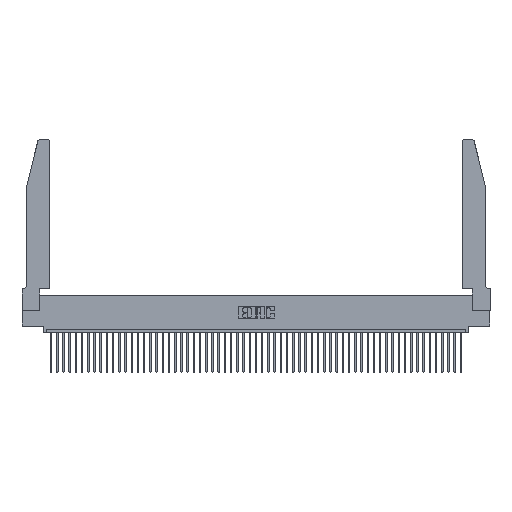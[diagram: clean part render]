
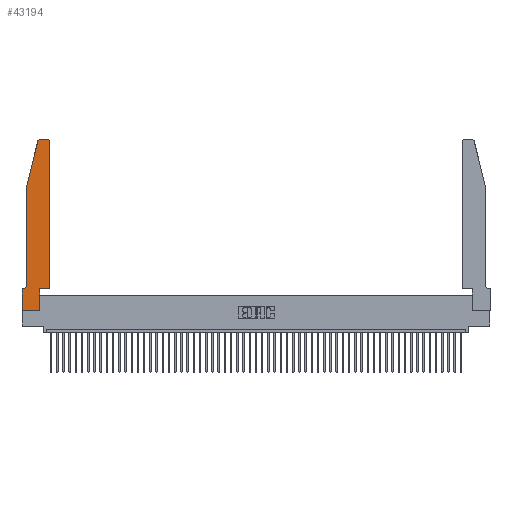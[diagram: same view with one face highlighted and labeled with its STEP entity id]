
A CAD part, top view. The second image highlights one B-rep face of the part: STEP entity #43194.
In plain terms, the highlighted planar face has unit normal (0, 0, 1).
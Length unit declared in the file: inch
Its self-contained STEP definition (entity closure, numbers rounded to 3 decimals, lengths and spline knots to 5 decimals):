
#188 = EDGE_LOOP ( 'NONE', ( #15539, #263, #4675, #17371, #25814, #16195, #5361, #44712, #41587, #32840, #48203, #21301 ) ) ;
#263 = ORIENTED_EDGE ( 'NONE', *, *, #28175, .T. ) ;
#366 = VERTEX_POINT ( 'NONE', #3941 ) ;
#711 = DIRECTION ( 'NONE',  ( 1., 0., 0. ) ) ;
#1036 = CARTESIAN_POINT ( 'NONE',  ( 0.4505, 0.35, 0.37 ) ) ;
#1436 = AXIS2_PLACEMENT_3D ( 'NONE', #32717, #16441, #5233 ) ;
#1506 = VERTEX_POINT ( 'NONE', #40229 ) ;
#2761 = CARTESIAN_POINT ( 'NONE',  ( 0.2865, 0.35, 0.37 ) ) ;
#3041 = VECTOR ( 'NONE', #23626, 39.37008 ) ;
#3048 = CARTESIAN_POINT ( 'NONE',  ( 0., 0.35, 0.37 ) ) ;
#3309 = VERTEX_POINT ( 'NONE', #19532 ) ;
#3941 = CARTESIAN_POINT ( 'NONE',  ( 0.2865, 0., 0.37 ) ) ;
#4309 = LINE ( 'NONE', #30593, #48179 ) ;
#4675 = ORIENTED_EDGE ( 'NONE', *, *, #12563, .T. ) ;
#5233 = DIRECTION ( 'NONE',  ( 1., 0., 0. ) ) ;
#5361 = ORIENTED_EDGE ( 'NONE', *, *, #14542, .T. ) ;
#6517 = LINE ( 'NONE', #10998, #42180 ) ;
#7146 = AXIS2_PLACEMENT_3D ( 'NONE', #3048, #35055, #39595 ) ;
#7967 = CARTESIAN_POINT ( 'NONE',  ( 0.2605, 2.75, 0.37 ) ) ;
#8789 = DIRECTION ( 'NONE',  ( 0., 1., 0. ) ) ;
#10096 = LINE ( 'NONE', #45011, #44548 ) ;
#10459 = DIRECTION ( 'NONE',  ( 0., 1., 0. ) ) ;
#10569 = AXIS2_PLACEMENT_3D ( 'NONE', #41142, #24911, #16986 ) ;
#10998 = CARTESIAN_POINT ( 'NONE',  ( 0.0755, 0.35, 0.37 ) ) ;
#11229 = CARTESIAN_POINT ( 'NONE',  ( 0.25487, 2.72718, 0.37 ) ) ;
#12563 = EDGE_CURVE ( 'NONE', #13031, #3309, #36550, .T. ) ;
#13031 = VERTEX_POINT ( 'NONE', #11229 ) ;
#13241 = EDGE_CURVE ( 'NONE', #15223, #44950, #6517, .T. ) ;
#13855 = LINE ( 'NONE', #7967, #19550 ) ;
#14542 = EDGE_CURVE ( 'NONE', #44950, #41553, #10096, .T. ) ;
#14568 = PLANE ( 'NONE',  #7146 ) ;
#15223 = VERTEX_POINT ( 'NONE', #27215 ) ;
#15321 = DIRECTION ( 'NONE',  ( -0.239, -0.971, 0. ) ) ;
#15539 = ORIENTED_EDGE ( 'NONE', *, *, #21559, .T. ) ;
#16195 = ORIENTED_EDGE ( 'NONE', *, *, #13241, .T. ) ;
#16441 = DIRECTION ( 'NONE',  ( 0., 0., 1. ) ) ;
#16543 = VECTOR ( 'NONE', #45865, 39.37008 ) ;
#16652 = VERTEX_POINT ( 'NONE', #2761 ) ;
#16986 = DIRECTION ( 'NONE',  ( -1., 0., 0. ) ) ;
#17343 = LINE ( 'NONE', #51008, #3041 ) ;
#17371 = ORIENTED_EDGE ( 'NONE', *, *, #26208, .T. ) ;
#17796 = CARTESIAN_POINT ( 'NONE',  ( 0.0755, 2., 0.37 ) ) ;
#18083 = VERTEX_POINT ( 'NONE', #34695 ) ;
#18189 = CARTESIAN_POINT ( 'NONE',  ( 0., 0.35, 0.37 ) ) ;
#19532 = CARTESIAN_POINT ( 'NONE',  ( 0.0755, 2., 0.37 ) ) ;
#19550 = VECTOR ( 'NONE', #44036, 39.37008 ) ;
#20001 = CIRCLE ( 'NONE', #10569, 0.07 ) ;
#20693 = DIRECTION ( 'NONE',  ( 0., 0., 1. ) ) ;
#21056 = VECTOR ( 'NONE', #8789, 39.37008 ) ;
#21301 = ORIENTED_EDGE ( 'NONE', *, *, #34798, .T. ) ;
#21559 = EDGE_CURVE ( 'NONE', #1506, #18083, #13855, .T. ) ;
#21628 = VERTEX_POINT ( 'NONE', #26570 ) ;
#22918 = EDGE_CURVE ( 'NONE', #25611, #15223, #20001, .T. ) ;
#23506 = CARTESIAN_POINT ( 'NONE',  ( 0.4505, 2.72, 0.37 ) ) ;
#23570 = LINE ( 'NONE', #43936, #39795 ) ;
#23626 = DIRECTION ( 'NONE',  ( 1., 0., 0. ) ) ;
#23788 = DIRECTION ( 'NONE',  ( -1., 0., 0. ) ) ;
#24079 = CARTESIAN_POINT ( 'NONE',  ( 0.0755, 2., 0.37 ) ) ;
#24690 = VECTOR ( 'NONE', #15321, 39.37008 ) ;
#24911 = DIRECTION ( 'NONE',  ( 0., 0., -1. ) ) ;
#25611 = VERTEX_POINT ( 'NONE', #25922 ) ;
#25814 = ORIENTED_EDGE ( 'NONE', *, *, #22918, .T. ) ;
#25922 = CARTESIAN_POINT ( 'NONE',  ( 0.0755, 0.42, 0.37 ) ) ;
#26208 = EDGE_CURVE ( 'NONE', #3309, #25611, #50506, .T. ) ;
#26570 = CARTESIAN_POINT ( 'NONE',  ( 0.4505, 0.35, 0.37 ) ) ;
#27215 = CARTESIAN_POINT ( 'NONE',  ( 0.0055, 0.35, 0.37 ) ) ;
#27835 = AXIS2_PLACEMENT_3D ( 'NONE', #32440, #20693, #711 ) ;
#28175 = EDGE_CURVE ( 'NONE', #18083, #13031, #44533, .T. ) ;
#29553 = DIRECTION ( 'NONE',  ( 0., -1., 0. ) ) ;
#30593 = CARTESIAN_POINT ( 'NONE',  ( 0.2865, 0.35, 0.37 ) ) ;
#31787 = LINE ( 'NONE', #1036, #21056 ) ;
#32440 = CARTESIAN_POINT ( 'NONE',  ( 0.284, 2.72, 0.37 ) ) ;
#32579 = EDGE_CURVE ( 'NONE', #21628, #35096, #31787, .T. ) ;
#32717 = CARTESIAN_POINT ( 'NONE',  ( 0.4205, 2.72, 0.37 ) ) ;
#32840 = ORIENTED_EDGE ( 'NONE', *, *, #39797, .T. ) ;
#34695 = CARTESIAN_POINT ( 'NONE',  ( 0.284, 2.75, 0.37 ) ) ;
#34798 = EDGE_CURVE ( 'NONE', #35096, #1506, #45306, .T. ) ;
#35055 = DIRECTION ( 'NONE',  ( 0., 0., 1. ) ) ;
#35096 = VERTEX_POINT ( 'NONE', #23506 ) ;
#35838 = DIRECTION ( 'NONE',  ( 1., 0., 0. ) ) ;
#36550 = LINE ( 'NONE', #24079, #24690 ) ;
#38585 = CARTESIAN_POINT ( 'NONE',  ( 0., 0., 0.37 ) ) ;
#39595 = DIRECTION ( 'NONE',  ( 1., 0., 0. ) ) ;
#39757 = EDGE_CURVE ( 'NONE', #366, #16652, #4309, .T. ) ;
#39795 = VECTOR ( 'NONE', #35838, 39.37008 ) ;
#39797 = EDGE_CURVE ( 'NONE', #16652, #21628, #17343, .T. ) ;
#40229 = CARTESIAN_POINT ( 'NONE',  ( 0.4205, 2.75, 0.37 ) ) ;
#41142 = CARTESIAN_POINT ( 'NONE',  ( 0.0055, 0.42, 0.37 ) ) ;
#41553 = VERTEX_POINT ( 'NONE', #38585 ) ;
#41587 = ORIENTED_EDGE ( 'NONE', *, *, #39757, .T. ) ;
#42180 = VECTOR ( 'NONE', #23788, 39.37008 ) ;
#43194 = ADVANCED_FACE ( 'NONE', ( #50967 ), #14568, .T. ) ;
#43936 = CARTESIAN_POINT ( 'NONE',  ( 0., 0., 0.37 ) ) ;
#44036 = DIRECTION ( 'NONE',  ( -1., 0., 0. ) ) ;
#44533 = CIRCLE ( 'NONE', #27835, 0.03 ) ;
#44548 = VECTOR ( 'NONE', #29553, 39.37008 ) ;
#44712 = ORIENTED_EDGE ( 'NONE', *, *, #45967, .T. ) ;
#44950 = VERTEX_POINT ( 'NONE', #18189 ) ;
#45011 = CARTESIAN_POINT ( 'NONE',  ( 0., 0., 0.37 ) ) ;
#45306 = CIRCLE ( 'NONE', #1436, 0.03 ) ;
#45865 = DIRECTION ( 'NONE',  ( 0., -1., 0. ) ) ;
#45967 = EDGE_CURVE ( 'NONE', #41553, #366, #23570, .T. ) ;
#48179 = VECTOR ( 'NONE', #10459, 39.37008 ) ;
#48203 = ORIENTED_EDGE ( 'NONE', *, *, #32579, .T. ) ;
#50506 = LINE ( 'NONE', #17796, #16543 ) ;
#50967 = FACE_OUTER_BOUND ( 'NONE', #188, .T. ) ;
#51008 = CARTESIAN_POINT ( 'NONE',  ( 0.4505, 0.35, 0.37 ) ) ;
